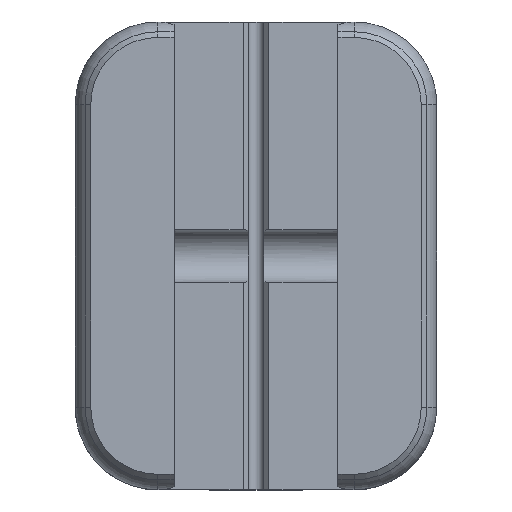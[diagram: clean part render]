
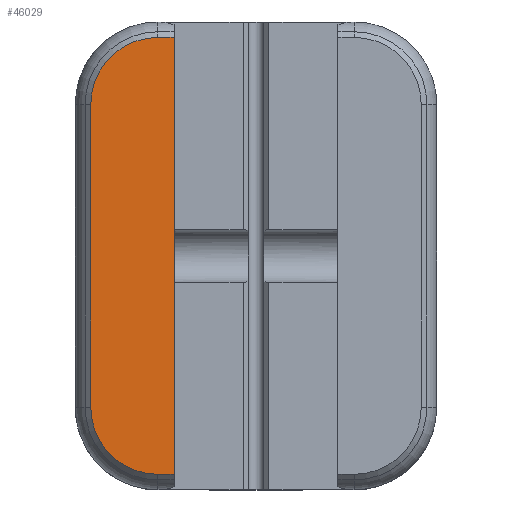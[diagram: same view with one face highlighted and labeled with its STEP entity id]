
A CAD part, top view. The second image highlights one B-rep face of the part: STEP entity #46029.
In plain terms, the highlighted planar face has unit normal (0, 0, 1).
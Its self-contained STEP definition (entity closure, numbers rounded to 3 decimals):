
#1075=CIRCLE('',#49578,6.5);
#1076=CIRCLE('',#49581,6.5);
#4065=FACE_OUTER_BOUND('',#7088,.T.);
#7088=EDGE_LOOP('',(#40098,#40099,#40100,#40101,#40102,#40103));
#12705=LINE('',#76770,#18350);
#12708=LINE('',#76778,#18353);
#12719=LINE('',#76805,#18364);
#12722=LINE('',#76810,#18367);
#18350=VECTOR('',#62223,10.);
#18353=VECTOR('',#62232,10.);
#18364=VECTOR('',#62261,10.);
#18367=VECTOR('',#62268,10.);
#21015=VERTEX_POINT('',#76762);
#21016=VERTEX_POINT('',#76764);
#21017=VERTEX_POINT('',#76768);
#21018=VERTEX_POINT('',#76772);
#21019=VERTEX_POINT('',#76776);
#21026=VERTEX_POINT('',#76804);
#27385=EDGE_CURVE('',#21015,#21016,#1075,.T.);
#27388=EDGE_CURVE('',#21017,#21015,#12705,.T.);
#27390=EDGE_CURVE('',#21018,#21017,#1076,.T.);
#27392=EDGE_CURVE('',#21019,#21018,#12708,.T.);
#27406=EDGE_CURVE('',#21016,#21026,#12719,.T.);
#27409=EDGE_CURVE('',#21026,#21019,#12722,.F.);
#40098=ORIENTED_EDGE('',*,*,#27406,.F.);
#40099=ORIENTED_EDGE('',*,*,#27385,.F.);
#40100=ORIENTED_EDGE('',*,*,#27388,.F.);
#40101=ORIENTED_EDGE('',*,*,#27390,.F.);
#40102=ORIENTED_EDGE('',*,*,#27392,.F.);
#40103=ORIENTED_EDGE('',*,*,#27409,.F.);
#43022=PLANE('',#49594);
#46029=ADVANCED_FACE('',(#4065),#43022,.F.);
#49578=AXIS2_PLACEMENT_3D('',#76765,#62217,#62218);
#49581=AXIS2_PLACEMENT_3D('',#76774,#62227,#62228);
#49594=AXIS2_PLACEMENT_3D('',#76812,#62270,#62271);
#62217=DIRECTION('center_axis',(0.,0.,
-1.));
#62218=DIRECTION('ref_axis',(-0.707,0.707,0.));
#62223=DIRECTION('',(0.,1.,0.));
#62227=DIRECTION('center_axis',(0.,0.,
-1.));
#62228=DIRECTION('ref_axis',(-0.707,-0.707,0.));
#62232=DIRECTION('',(-1.,0.,0.));
#62261=DIRECTION('',(1.,0.,0.));
#62268=DIRECTION('',(0.,1.,0.));
#62270=DIRECTION('center_axis',(0.,0.,
-1.));
#62271=DIRECTION('ref_axis',(1.,0.,0.));
#76762=CARTESIAN_POINT('',(-16.,69.653,-24.354));
#76764=CARTESIAN_POINT('',(-9.5,76.153,-24.354));
#76765=CARTESIAN_POINT('Origin',(-9.5,69.653,-24.354));
#76768=CARTESIAN_POINT('',(-16.,40.355,-24.354));
#76770=CARTESIAN_POINT('',(-16.,69.903,-24.354));
#76772=CARTESIAN_POINT('',(-9.5,33.855,-24.354));
#76774=CARTESIAN_POINT('Origin',(-9.5,40.355,-24.354));
#76776=CARTESIAN_POINT('',(-7.936,33.855,-24.354));
#76778=CARTESIAN_POINT('',(-10.135,33.855,-24.354));
#76804=CARTESIAN_POINT('',(-7.936,76.153,-24.354));
#76805=CARTESIAN_POINT('',(-10.135,76.153,-24.354));
#76810=CARTESIAN_POINT('',(-7.936,42.504,-24.354));
#76812=CARTESIAN_POINT('Origin',(-20.269,69.903,-24.354));
